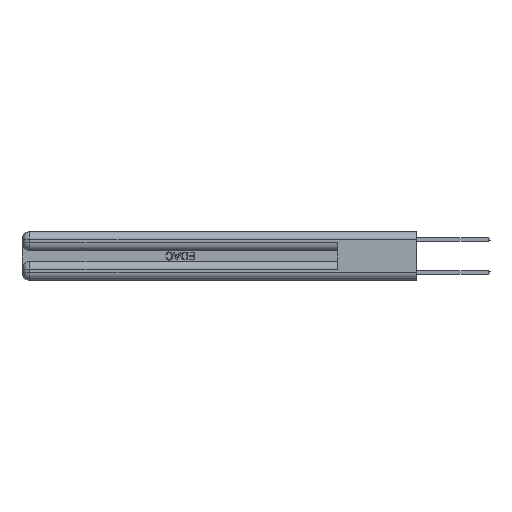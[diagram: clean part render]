
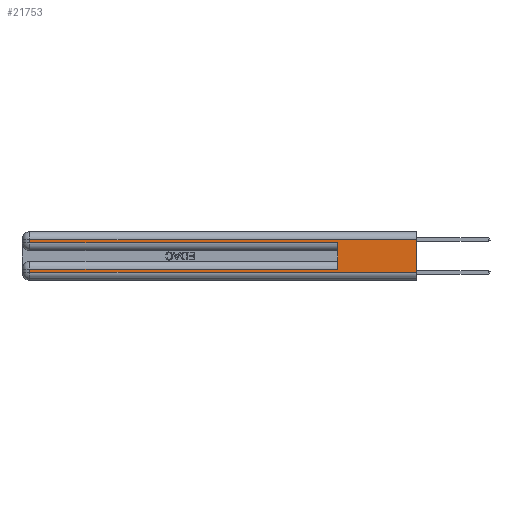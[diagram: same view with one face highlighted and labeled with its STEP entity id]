
A CAD part, left-side view. The second image highlights one B-rep face of the part: STEP entity #21753.
In plain terms, the highlighted planar face has unit normal (-1, 0, 0).
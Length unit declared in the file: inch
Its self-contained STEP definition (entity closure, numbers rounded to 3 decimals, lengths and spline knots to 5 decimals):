
#1114 = LINE ( 'NONE', #19779, #22796 ) ;
#1428 = VERTEX_POINT ( 'NONE', #19531 ) ;
#1606 = EDGE_LOOP ( 'NONE', ( #34386, #17447, #32819, #23019, #31556, #16218, #21415, #17638 ) ) ;
#2362 = CARTESIAN_POINT ( 'NONE',  ( 0., 0., 0.285 ) ) ;
#3457 = LINE ( 'NONE', #33317, #10880 ) ;
#3497 = CARTESIAN_POINT ( 'NONE',  ( 0., 0., 0.31 ) ) ;
#4364 = FACE_OUTER_BOUND ( 'NONE', #1606, .T. ) ;
#4496 = DIRECTION ( 'NONE',  ( 0., -1., 0. ) ) ;
#5258 = CARTESIAN_POINT ( 'NONE',  ( 0., 2.94, 0.37 ) ) ;
#5279 = EDGE_CURVE ( 'NONE', #8309, #6172, #13336, .T. ) ;
#5310 = DIRECTION ( 'NONE',  ( 0., 1., 0. ) ) ;
#5621 = CARTESIAN_POINT ( 'NONE',  ( 0., 2.94, 0.085 ) ) ;
#6172 = VERTEX_POINT ( 'NONE', #5621 ) ;
#7667 = LINE ( 'NONE', #2362, #30520 ) ;
#8309 = VERTEX_POINT ( 'NONE', #24724 ) ;
#9356 = DIRECTION ( 'NONE',  ( 1., 0., 0. ) ) ;
#9533 = EDGE_CURVE ( 'NONE', #1428, #14732, #7667, .T. ) ;
#9748 = VECTOR ( 'NONE', #5310, 39.37008 ) ;
#10420 = DIRECTION ( 'NONE',  ( 0., 0., -1. ) ) ;
#10880 = VECTOR ( 'NONE', #27439, 39.37008 ) ;
#11609 = EDGE_CURVE ( 'NONE', #26877, #12612, #25168, .T. ) ;
#11659 = CARTESIAN_POINT ( 'NONE',  ( 0., 0., 0.06 ) ) ;
#11964 = DIRECTION ( 'NONE',  ( 0., 0., -1. ) ) ;
#12612 = VERTEX_POINT ( 'NONE', #18783 ) ;
#13336 = LINE ( 'NONE', #22409, #34410 ) ;
#13433 = VECTOR ( 'NONE', #10420, 39.37008 ) ;
#14732 = VERTEX_POINT ( 'NONE', #33935 ) ;
#15341 = AXIS2_PLACEMENT_3D ( 'NONE', #23216, #9356, #25346 ) ;
#16218 = ORIENTED_EDGE ( 'NONE', *, *, #5279, .T. ) ;
#17447 = ORIENTED_EDGE ( 'NONE', *, *, #24954, .T. ) ;
#17638 = ORIENTED_EDGE ( 'NONE', *, *, #11609, .T. ) ;
#18783 = CARTESIAN_POINT ( 'NONE',  ( 0., 0., 0.06 ) ) ;
#19297 = VECTOR ( 'NONE', #22507, 39.37008 ) ;
#19446 = LINE ( 'NONE', #32962, #20304 ) ;
#19531 = CARTESIAN_POINT ( 'NONE',  ( 0., 2.94, 0.285 ) ) ;
#19554 = CARTESIAN_POINT ( 'NONE',  ( 0., 2.94, 0.06 ) ) ;
#19779 = CARTESIAN_POINT ( 'NONE',  ( 0., 0., 0.37 ) ) ;
#20304 = VECTOR ( 'NONE', #27432, 39.37008 ) ;
#21415 = ORIENTED_EDGE ( 'NONE', *, *, #25447, .T. ) ;
#21483 = LINE ( 'NONE', #3497, #9748 ) ;
#21753 = ADVANCED_FACE ( 'NONE', ( #4364 ), #31550, .F. ) ;
#22409 = CARTESIAN_POINT ( 'NONE',  ( 0., 0., 0.085 ) ) ;
#22505 = CARTESIAN_POINT ( 'NONE',  ( 0., 0., 0.31 ) ) ;
#22507 = DIRECTION ( 'NONE',  ( 0., -1., 0. ) ) ;
#22709 = CARTESIAN_POINT ( 'NONE',  ( 0., 2.94, 0.31 ) ) ;
#22796 = VECTOR ( 'NONE', #11964, 39.37008 ) ;
#22952 = EDGE_CURVE ( 'NONE', #34221, #12612, #1114, .T. ) ;
#23019 = ORIENTED_EDGE ( 'NONE', *, *, #9533, .T. ) ;
#23216 = CARTESIAN_POINT ( 'NONE',  ( 0., 0., 0.37 ) ) ;
#24724 = CARTESIAN_POINT ( 'NONE',  ( 0., 0.6, 0.085 ) ) ;
#24954 = EDGE_CURVE ( 'NONE', #34221, #31263, #21483, .T. ) ;
#25168 = LINE ( 'NONE', #11659, #19297 ) ;
#25346 = DIRECTION ( 'NONE',  ( 0., 0., -1. ) ) ;
#25447 = EDGE_CURVE ( 'NONE', #6172, #26877, #3457, .T. ) ;
#26877 = VERTEX_POINT ( 'NONE', #19554 ) ;
#27114 = LINE ( 'NONE', #5258, #13433 ) ;
#27432 = DIRECTION ( 'NONE',  ( 0., 0., 1. ) ) ;
#27439 = DIRECTION ( 'NONE',  ( 0., 0., -1. ) ) ;
#30048 = DIRECTION ( 'NONE',  ( 0., 1., 0. ) ) ;
#30520 = VECTOR ( 'NONE', #4496, 39.37008 ) ;
#30885 = EDGE_CURVE ( 'NONE', #8309, #14732, #19446, .T. ) ;
#31263 = VERTEX_POINT ( 'NONE', #22709 ) ;
#31550 = PLANE ( 'NONE',  #15341 ) ;
#31556 = ORIENTED_EDGE ( 'NONE', *, *, #30885, .F. ) ;
#32808 = EDGE_CURVE ( 'NONE', #31263, #1428, #27114, .T. ) ;
#32819 = ORIENTED_EDGE ( 'NONE', *, *, #32808, .T. ) ;
#32962 = CARTESIAN_POINT ( 'NONE',  ( 0., 0.6, 0.145 ) ) ;
#33317 = CARTESIAN_POINT ( 'NONE',  ( 0., 2.94, 0.37 ) ) ;
#33935 = CARTESIAN_POINT ( 'NONE',  ( 0., 0.6, 0.285 ) ) ;
#34221 = VERTEX_POINT ( 'NONE', #22505 ) ;
#34386 = ORIENTED_EDGE ( 'NONE', *, *, #22952, .F. ) ;
#34410 = VECTOR ( 'NONE', #30048, 39.37008 ) ;
